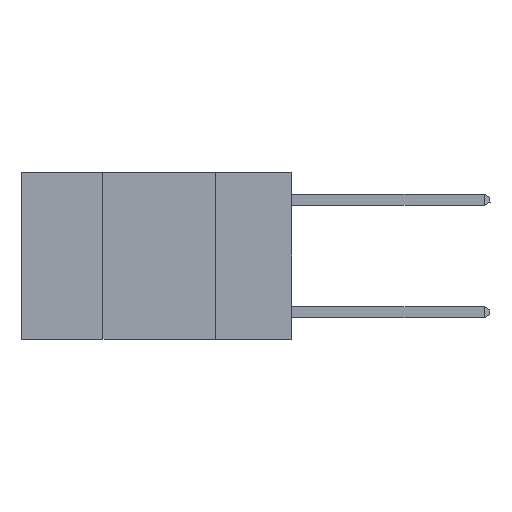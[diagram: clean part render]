
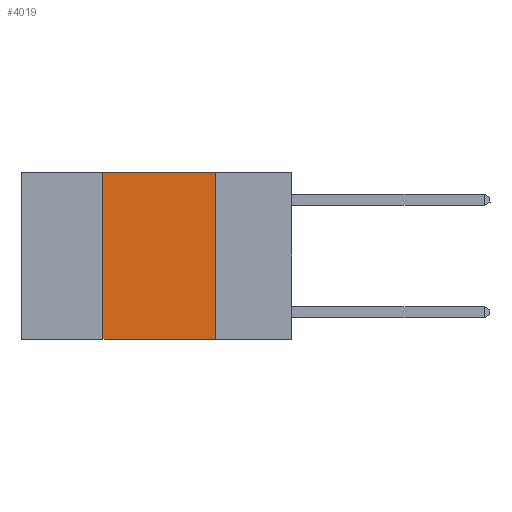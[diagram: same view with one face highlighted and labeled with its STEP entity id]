
A CAD part, left-side view. The second image highlights one B-rep face of the part: STEP entity #4019.
In plain terms, the highlighted planar face has unit normal (-1, 0, 0).
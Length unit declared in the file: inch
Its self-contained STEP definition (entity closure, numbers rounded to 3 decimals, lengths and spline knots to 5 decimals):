
#102 = LINE ( 'NONE', #10467, #494 ) ;
#365 = ORIENTED_EDGE ( 'NONE', *, *, #9160, .F. ) ;
#423 = DIRECTION ( 'NONE',  ( 0., 0., -1. ) ) ;
#471 = VECTOR ( 'NONE', #6094, 39.37008 ) ;
#494 = VECTOR ( 'NONE', #3000, 39.37008 ) ;
#973 = DIRECTION ( 'NONE',  ( 0., -1., 0. ) ) ;
#1227 = VECTOR ( 'NONE', #12054, 39.37008 ) ;
#1675 = ORIENTED_EDGE ( 'NONE', *, *, #9202, .T. ) ;
#1809 = EDGE_CURVE ( 'NONE', #2609, #6790, #102, .T. ) ;
#2609 = VERTEX_POINT ( 'NONE', #15236 ) ;
#2888 = ORIENTED_EDGE ( 'NONE', *, *, #3419, .F. ) ;
#3000 = DIRECTION ( 'NONE',  ( 0., 0., -1. ) ) ;
#3309 = VERTEX_POINT ( 'NONE', #11810 ) ;
#3419 = EDGE_CURVE ( 'NONE', #3309, #2609, #15551, .T. ) ;
#4019 = ADVANCED_FACE ( 'NONE', ( #6541 ), #12788, .F. ) ;
#4833 = CARTESIAN_POINT ( 'NONE',  ( 0., 0.6, -0.37 ) ) ;
#6094 = DIRECTION ( 'NONE',  ( 0., -1., 0. ) ) ;
#6183 = ORIENTED_EDGE ( 'NONE', *, *, #1809, .F. ) ;
#6349 = VECTOR ( 'NONE', #973, 39.37008 ) ;
#6541 = FACE_OUTER_BOUND ( 'NONE', #9575, .T. ) ;
#6561 = AXIS2_PLACEMENT_3D ( 'NONE', #14948, #8062, #423 ) ;
#6790 = VERTEX_POINT ( 'NONE', #14625 ) ;
#8062 = DIRECTION ( 'NONE',  ( 1., 0., 0. ) ) ;
#9160 = EDGE_CURVE ( 'NONE', #14676, #3309, #11250, .T. ) ;
#9202 = EDGE_CURVE ( 'NONE', #14676, #6790, #13869, .T. ) ;
#9575 = EDGE_LOOP ( 'NONE', ( #6183, #2888, #365, #1675 ) ) ;
#10467 = CARTESIAN_POINT ( 'NONE',  ( 0., 0.17, 0. ) ) ;
#10831 = CARTESIAN_POINT ( 'NONE',  ( 0., 0.42, 0. ) ) ;
#11250 = LINE ( 'NONE', #10831, #1227 ) ;
#11594 = CARTESIAN_POINT ( 'NONE',  ( 0., 0.42, -0.37 ) ) ;
#11810 = CARTESIAN_POINT ( 'NONE',  ( 0., 0.42, 0. ) ) ;
#12054 = DIRECTION ( 'NONE',  ( 0., 0., 1. ) ) ;
#12788 = PLANE ( 'NONE',  #6561 ) ;
#13869 = LINE ( 'NONE', #4833, #471 ) ;
#14625 = CARTESIAN_POINT ( 'NONE',  ( 0., 0.17, -0.37 ) ) ;
#14676 = VERTEX_POINT ( 'NONE', #11594 ) ;
#14948 = CARTESIAN_POINT ( 'NONE',  ( 0., 0.6, 0. ) ) ;
#15236 = CARTESIAN_POINT ( 'NONE',  ( 0., 0.17, 0. ) ) ;
#15443 = CARTESIAN_POINT ( 'NONE',  ( 0., 0.6, 0. ) ) ;
#15551 = LINE ( 'NONE', #15443, #6349 ) ;
